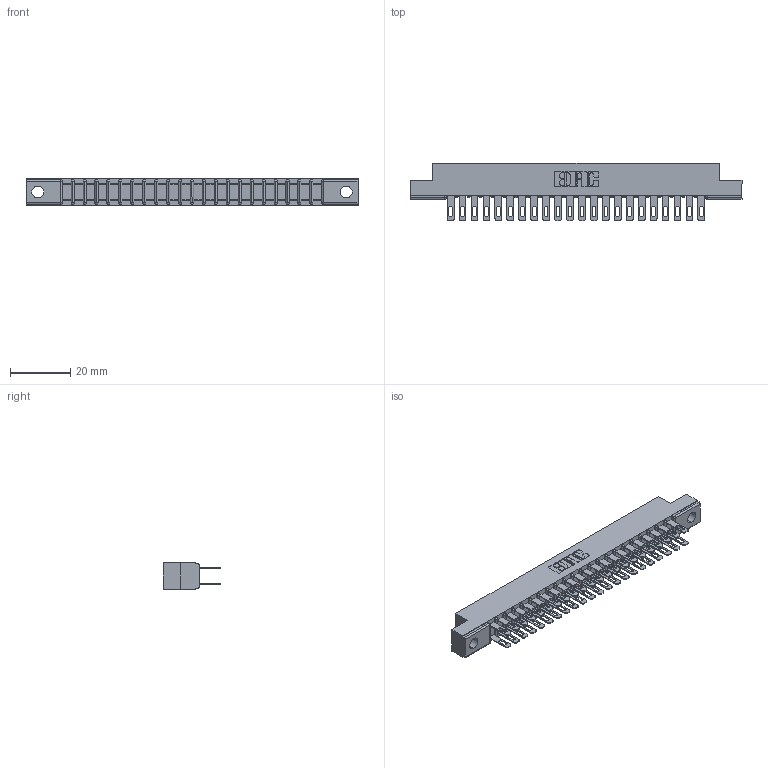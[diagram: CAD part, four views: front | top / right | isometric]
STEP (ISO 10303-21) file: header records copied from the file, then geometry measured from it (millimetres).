
FILE_DESCRIPTION (( 'STEP AP203' ), '1' );
FILE_NAME ('357-044-500-202.STEP', '2018-08-11T11:56:11', ( '' ), ( '' ), 'SwSTEP 2.0', 'SolidWorks 2016', '' );
FILE_SCHEMA (( 'CONFIG_CONTROL_DESIGN' ));
Length unit declared in the file: inch
Products named in the file (3): 307 Part_.128 Dia Mounting Holes; 307-290-001_500; 357-044-500-202
Assembly tree (45 placements, depth 2):
  357-044-500-202
    307 Part_.128 Dia Mounting Holes
    307-290-001_500  x44
Bounding box: 110.19 x 19.18 x 8.71 mm (x, y, z)
Volume: 7245.5 mm3; surface area: 13343.6 mm2
Topology: 45 solids, 45 shells, 2165 faces, 6043 edges, 3906 vertices
Faces by surface type: plane 1390, cylinder 729, sphere 46
Entity records: 22006 total; most frequent: CARTESIAN_POINT 3602, ORIENTED_EDGE 3566, DIRECTION 3539, EDGE_CURVE 1783, LINE 1357, VECTOR 1357, VERTEX_POINT 1154, AXIS2_PLACEMENT_3D 1091
